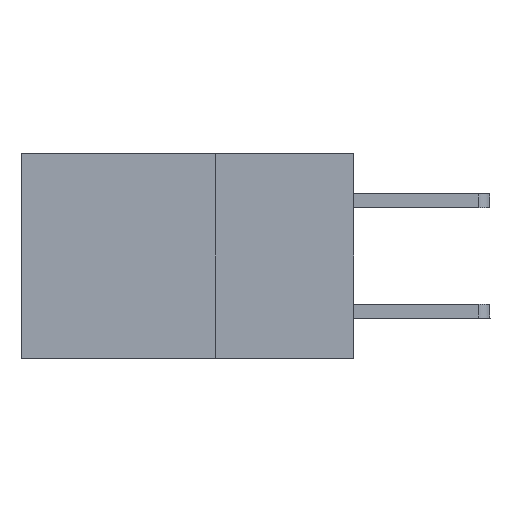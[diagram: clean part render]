
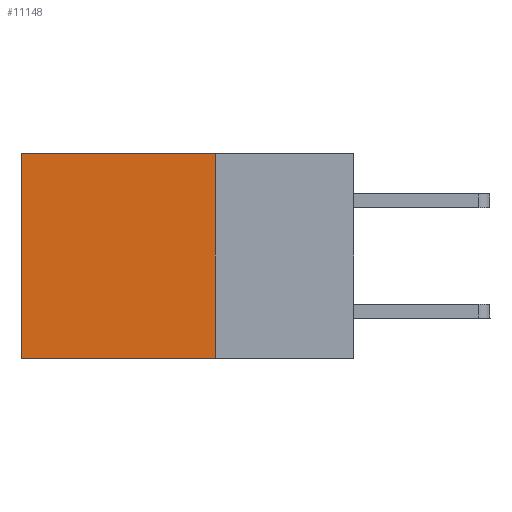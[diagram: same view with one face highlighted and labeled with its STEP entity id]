
A CAD part, left-side view. The second image highlights one B-rep face of the part: STEP entity #11148.
In plain terms, the highlighted planar face has unit normal (-1, 0, 0).
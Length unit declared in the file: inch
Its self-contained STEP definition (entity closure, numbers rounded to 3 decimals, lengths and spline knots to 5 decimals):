
#892 = EDGE_CURVE ( 'NONE', #14189, #3094, #9543, .T. ) ;
#1002 = EDGE_CURVE ( 'NONE', #2815, #3094, #2109, .T. ) ;
#1715 = VECTOR ( 'NONE', #2084, 39.37008 ) ;
#2013 = CARTESIAN_POINT ( 'NONE',  ( 0.2875, 0.25, 0. ) ) ;
#2084 = DIRECTION ( 'NONE',  ( 0., 0., -1. ) ) ;
#2109 = LINE ( 'NONE', #6642, #2358 ) ;
#2358 = VECTOR ( 'NONE', #14393, 39.37008 ) ;
#2815 = VERTEX_POINT ( 'NONE', #4541 ) ;
#3094 = VERTEX_POINT ( 'NONE', #6535 ) ;
#3233 = LINE ( 'NONE', #14617, #9526 ) ;
#3618 = AXIS2_PLACEMENT_3D ( 'NONE', #7501, #6034, #11066 ) ;
#4541 = CARTESIAN_POINT ( 'NONE',  ( 0.2875, 0.25, -0.37 ) ) ;
#5272 = PLANE ( 'NONE',  #3618 ) ;
#6034 = DIRECTION ( 'NONE',  ( 1., 0., 0. ) ) ;
#6535 = CARTESIAN_POINT ( 'NONE',  ( 0.2875, 0.6, -0.37 ) ) ;
#6642 = CARTESIAN_POINT ( 'NONE',  ( 0.2875, 0.25, -0.37 ) ) ;
#6774 = ORIENTED_EDGE ( 'NONE', *, *, #1002, .F. ) ;
#7173 = VERTEX_POINT ( 'NONE', #2013 ) ;
#7388 = CARTESIAN_POINT ( 'NONE',  ( 0.2875, 0.6, 0. ) ) ;
#7441 = ORIENTED_EDGE ( 'NONE', *, *, #9596, .F. ) ;
#7501 = CARTESIAN_POINT ( 'NONE',  ( 0.2875, 0.25, 0. ) ) ;
#7616 = DIRECTION ( 'NONE',  ( 0., 1., 0. ) ) ;
#8338 = FACE_OUTER_BOUND ( 'NONE', #10142, .T. ) ;
#8877 = CARTESIAN_POINT ( 'NONE',  ( 0.2875, 0.6, 0. ) ) ;
#9219 = ORIENTED_EDGE ( 'NONE', *, *, #892, .T. ) ;
#9526 = VECTOR ( 'NONE', #7616, 39.37008 ) ;
#9543 = LINE ( 'NONE', #7388, #11378 ) ;
#9596 = EDGE_CURVE ( 'NONE', #7173, #2815, #12280, .T. ) ;
#10142 = EDGE_LOOP ( 'NONE', ( #9219, #6774, #7441, #12716 ) ) ;
#10245 = CARTESIAN_POINT ( 'NONE',  ( 0.2875, 0.25, 0. ) ) ;
#10549 = EDGE_CURVE ( 'NONE', #7173, #14189, #3233, .T. ) ;
#11066 = DIRECTION ( 'NONE',  ( 0., 0., -1. ) ) ;
#11148 = ADVANCED_FACE ( 'NONE', ( #8338 ), #5272, .F. ) ;
#11378 = VECTOR ( 'NONE', #14022, 39.37008 ) ;
#12280 = LINE ( 'NONE', #10245, #1715 ) ;
#12716 = ORIENTED_EDGE ( 'NONE', *, *, #10549, .T. ) ;
#14022 = DIRECTION ( 'NONE',  ( 0., 0., -1. ) ) ;
#14189 = VERTEX_POINT ( 'NONE', #8877 ) ;
#14393 = DIRECTION ( 'NONE',  ( 0., 1., 0. ) ) ;
#14617 = CARTESIAN_POINT ( 'NONE',  ( 0.2875, 0.25, 0. ) ) ;
